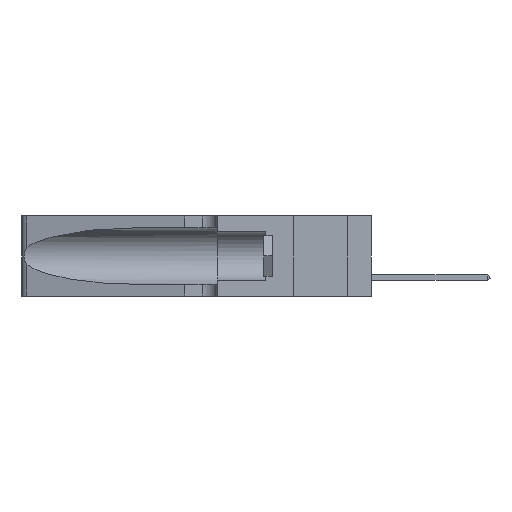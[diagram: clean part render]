
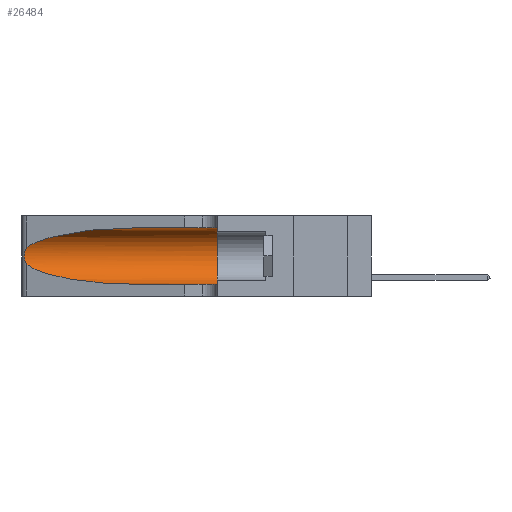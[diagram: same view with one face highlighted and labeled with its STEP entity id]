
A CAD part, left-side view. The second image highlights one B-rep face of the part: STEP entity #26484.
In plain terms, the highlighted cylindrical face has radius 3.308 mm (diameter 6.617 mm), a partial arc.
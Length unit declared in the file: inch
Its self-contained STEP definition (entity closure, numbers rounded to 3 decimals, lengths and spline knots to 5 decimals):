
#794 = DIRECTION ( 'NONE',  ( 0., -1., 0. ) ) ;
#2887 = VERTEX_POINT ( 'NONE', #25936 ) ;
#3342 = ORIENTED_EDGE ( 'NONE', *, *, #29236, .T. ) ;
#3535 = CARTESIAN_POINT ( 'NONE',  ( 0.25487, 1.22718, 0.22369 ) ) ;
#3717 = CARTESIAN_POINT ( 'NONE',  ( 0.26018, 1.23835, 0.19895 ) ) ;
#3845 = FACE_OUTER_BOUND ( 'NONE', #19785, .T. ) ;
#3869 = CARTESIAN_POINT ( 'NONE',  ( 0.26017, 1.23833, 0.17102 ) ) ;
#4004 = CARTESIAN_POINT ( 'NONE',  ( 0.25789, 1.23486, 0.15765 ) ) ;
#4065 = CARTESIAN_POINT ( 'NONE',  ( 0.2373, 1.15595, 0.28018 ) ) ;
#4993 = EDGE_CURVE ( 'NONE', #35677, #42179, #12513, .T. ) ;
#5034 = CARTESIAN_POINT ( 'NONE',  ( 0.1305, 0.35, 0.185 ) ) ;
#6182 = ORIENTED_EDGE ( 'NONE', *, *, #17461, .T. ) ;
#6531 = ORIENTED_EDGE ( 'NONE', *, *, #9420, .F. ) ;
#7075 = CARTESIAN_POINT ( 'NONE',  ( 0.26075, 1.23896, 0.19203 ) ) ;
#8330 = EDGE_CURVE ( 'NONE', #15598, #39570, #37957, .T. ) ;
#8349 = AXIS2_PLACEMENT_3D ( 'NONE', #5034, #11295, #21024 ) ;
#8774 = CARTESIAN_POINT ( 'NONE',  ( 0.25487, 1.22718, 0.14631 ) ) ;
#9420 = EDGE_CURVE ( 'NONE', #42179, #2887, #30288, .T. ) ;
#11022 = CARTESIAN_POINT ( 'NONE',  ( 0.1305, 1.61858, 0.31525 ) ) ;
#11295 = DIRECTION ( 'NONE',  ( 0., 1., 0. ) ) ;
#11838 = DIRECTION ( 'NONE',  ( 0., -1., 0. ) ) ;
#12329 = CARTESIAN_POINT ( 'NONE',  ( 0.1305, 0.35, 0.31525 ) ) ;
#12513 = LINE ( 'NONE', #11022, #13968 ) ;
#12558 = DIRECTION ( 'NONE',  ( 0., 0., -1. ) ) ;
#13968 = VECTOR ( 'NONE', #17862, 39.37008 ) ;
#15598 = VERTEX_POINT ( 'NONE', #8774 ) ;
#16352 = EDGE_CURVE ( 'NONE', #18210, #15598, #42569, .T. ) ;
#16773 = ORIENTED_EDGE ( 'NONE', *, *, #4993, .F. ) ;
#17431 = CARTESIAN_POINT ( 'NONE',  ( 0.1305, 1.61858, 0.05475 ) ) ;
#17461 = EDGE_CURVE ( 'NONE', #35677, #18210, #27018, .T. ) ;
#17729 = CARTESIAN_POINT ( 'NONE',  ( 0.2373, 1.15595, 0.08982 ) ) ;
#17862 = DIRECTION ( 'NONE',  ( 0., -1., 0. ) ) ;
#18210 = VERTEX_POINT ( 'NONE', #23532 ) ;
#18901 = LINE ( 'NONE', #17431, #26729 ) ;
#19785 = EDGE_LOOP ( 'NONE', ( #6182, #30090, #25013, #3342, #6531, #16773 ) ) ;
#20600 = CARTESIAN_POINT ( 'NONE',  ( 0.25856, 1.23593, 0.16098 ) ) ;
#21024 = DIRECTION ( 'NONE',  ( 0., 0., 1. ) ) ;
#21878 = CARTESIAN_POINT ( 'NONE',  ( 0.1305, 0.72297, 0.05475 ) ) ;
#23267 = CARTESIAN_POINT ( 'NONE',  ( 0.25854, 1.2359, 0.20912 ) ) ;
#23447 = CARTESIAN_POINT ( 'NONE',  ( 0.18966, 0.96281, 0.31525 ) ) ;
#23532 = CARTESIAN_POINT ( 'NONE',  ( 0.25487, 1.22718, 0.22369 ) ) ;
#25013 = ORIENTED_EDGE ( 'NONE', *, *, #8330, .T. ) ;
#25049 = CARTESIAN_POINT ( 'NONE',  ( 0.1305, 1.61858, 0.185 ) ) ;
#25643 = CARTESIAN_POINT ( 'NONE',  ( 0.25487, 1.22718, 0.22369 ) ) ;
#25936 = CARTESIAN_POINT ( 'NONE',  ( 0.1305, 0.35, 0.05475 ) ) ;
#26239 = CARTESIAN_POINT ( 'NONE',  ( 0.25787, 1.23484, 0.2124 ) ) ;
#26484 = ADVANCED_FACE ( 'NONE', ( #3845 ), #39354, .F. ) ;
#26527 = CARTESIAN_POINT ( 'NONE',  ( 0.25639, 1.23184, 0.21858 ) ) ;
#26729 = VECTOR ( 'NONE', #794, 39.37008 ) ;
#27018 =( BOUNDED_CURVE ( )  B_SPLINE_CURVE ( 3, ( #37123, #23447, #4065, #3535 ),
 .UNSPECIFIED., .F., .F. ) 
 B_SPLINE_CURVE_WITH_KNOTS ( ( 4, 4 ),
 ( 1.5708, 2.84003 ),
 .UNSPECIFIED. ) 
 CURVE ( )  GEOMETRIC_REPRESENTATION_ITEM ( )  RATIONAL_B_SPLINE_CURVE ( ( 1., 0.87, 0.87, 1. ) ) 
 REPRESENTATION_ITEM ( '' )  );
#27606 = CARTESIAN_POINT ( 'NONE',  ( 0.25487, 1.22718, 0.14631 ) ) ;
#27915 = CARTESIAN_POINT ( 'NONE',  ( 0.25555, 1.22993, 0.14849 ) ) ;
#29236 = EDGE_CURVE ( 'NONE', #39570, #2887, #18901, .T. ) ;
#30090 = ORIENTED_EDGE ( 'NONE', *, *, #16352, .T. ) ;
#30288 = CIRCLE ( 'NONE', #8349, 0.13025 ) ;
#31917 = CARTESIAN_POINT ( 'NONE',  ( 0.1305, 0.72297, 0.31525 ) ) ;
#34010 = CARTESIAN_POINT ( 'NONE',  ( 0.25639, 1.23186, 0.15144 ) ) ;
#35677 = VERTEX_POINT ( 'NONE', #31917 ) ;
#37123 = CARTESIAN_POINT ( 'NONE',  ( 0.1305, 0.72297, 0.31525 ) ) ;
#37699 = CARTESIAN_POINT ( 'NONE',  ( 0.25487, 1.22718, 0.14631 ) ) ;
#37957 =( BOUNDED_CURVE ( )  B_SPLINE_CURVE ( 3, ( #37699, #17729, #41184, #41030 ),
 .UNSPECIFIED., .F., .T. ) 
 B_SPLINE_CURVE_WITH_KNOTS ( ( 4, 4 ),
 ( 3.44316, 4.71239 ),
 .UNSPECIFIED. ) 
 CURVE ( )  GEOMETRIC_REPRESENTATION_ITEM ( )  RATIONAL_B_SPLINE_CURVE ( ( 1., 0.87, 0.87, 1. ) ) 
 REPRESENTATION_ITEM ( '' )  );
#39354 = CYLINDRICAL_SURFACE ( 'NONE', #40824, 0.13025 ) ;
#39570 = VERTEX_POINT ( 'NONE', #21878 ) ;
#40426 = CARTESIAN_POINT ( 'NONE',  ( 0.26075, 1.23896, 0.178 ) ) ;
#40824 = AXIS2_PLACEMENT_3D ( 'NONE', #25049, #11838, #12558 ) ;
#41030 = CARTESIAN_POINT ( 'NONE',  ( 0.1305, 0.72297, 0.05475 ) ) ;
#41184 = CARTESIAN_POINT ( 'NONE',  ( 0.18966, 0.96281, 0.05475 ) ) ;
#42179 = VERTEX_POINT ( 'NONE', #12329 ) ;
#42408 = CARTESIAN_POINT ( 'NONE',  ( 0.25555, 1.22994, 0.2215 ) ) ;
#42569 = B_SPLINE_CURVE_WITH_KNOTS ( 'NONE', 3,
 ( #25643, #42408, #26527, #26239, #23267, #3717, #7075, #40426, #3869, #20600, #4004, #34010, #27915, #27606 ),
 .UNSPECIFIED., .F., .F.,
 ( 4, 2, 2, 2, 2, 2, 4 ),
 ( 0., 0.00027, 0.00053, 0.00107, 0.0016, 0.00187, 0.00214 ),
 .UNSPECIFIED. ) ;
